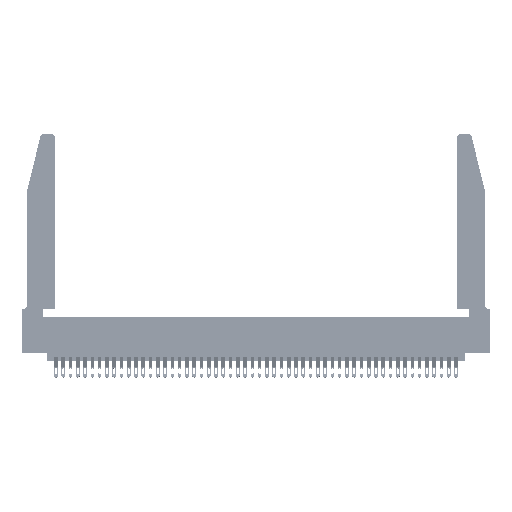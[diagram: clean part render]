
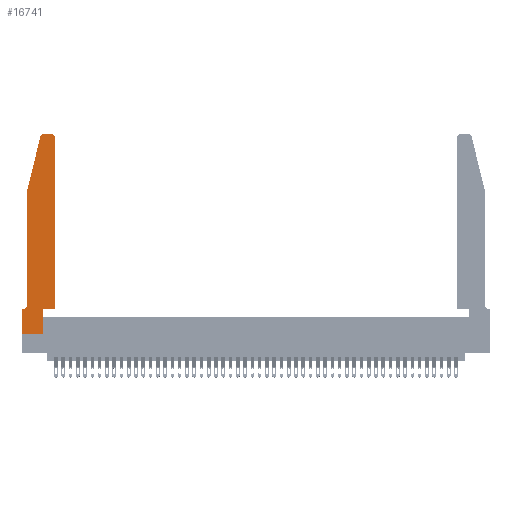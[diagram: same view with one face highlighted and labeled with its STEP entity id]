
A CAD part, top view. The second image highlights one B-rep face of the part: STEP entity #16741.
In plain terms, the highlighted planar face has unit normal (0, 0, 1).
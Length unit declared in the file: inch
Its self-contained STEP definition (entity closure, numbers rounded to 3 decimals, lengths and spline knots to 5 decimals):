
#298 = ORIENTED_EDGE ( 'NONE', *, *, #28404, .T. ) ;
#1066 = DIRECTION ( 'NONE',  ( 0., 0., -1. ) ) ;
#1741 = CARTESIAN_POINT ( 'NONE',  ( 0.0755, 2., 0.37 ) ) ;
#4132 = EDGE_CURVE ( 'NONE', #17867, #7614, #18595, .T. ) ;
#4492 = AXIS2_PLACEMENT_3D ( 'NONE', #38347, #20218, #45527 ) ;
#4777 = VECTOR ( 'NONE', #9166, 39.37008 ) ;
#5422 = CARTESIAN_POINT ( 'NONE',  ( 0.0755, 2., 0.37 ) ) ;
#5758 = LINE ( 'NONE', #1741, #31540 ) ;
#5837 = CIRCLE ( 'NONE', #22130, 0.03 ) ;
#6157 = EDGE_CURVE ( 'NONE', #44111, #42202, #5837, .T. ) ;
#6162 = DIRECTION ( 'NONE',  ( 1., 0., 0. ) ) ;
#6697 = ORIENTED_EDGE ( 'NONE', *, *, #16941, .T. ) ;
#7207 = CARTESIAN_POINT ( 'NONE',  ( 0.2605, 2.75, 0.37 ) ) ;
#7307 = CARTESIAN_POINT ( 'NONE',  ( 0., 0., 0.37 ) ) ;
#7614 = VERTEX_POINT ( 'NONE', #37270 ) ;
#7860 = VERTEX_POINT ( 'NONE', #38351 ) ;
#8932 = DIRECTION ( 'NONE',  ( 0., 1., 0. ) ) ;
#9166 = DIRECTION ( 'NONE',  ( -0.239, -0.971, 0. ) ) ;
#9358 = EDGE_CURVE ( 'NONE', #42269, #7860, #24771, .T. ) ;
#9392 = VECTOR ( 'NONE', #27850, 39.37008 ) ;
#13150 = CARTESIAN_POINT ( 'NONE',  ( 0.0755, 0.35, 0.37 ) ) ;
#13157 = VECTOR ( 'NONE', #36526, 39.37008 ) ;
#13175 = EDGE_CURVE ( 'NONE', #7614, #32033, #39189, .T. ) ;
#13488 = DIRECTION ( 'NONE',  ( 0., 0., 1. ) ) ;
#14235 = CARTESIAN_POINT ( 'NONE',  ( 0.2865, 0.35, 0.37 ) ) ;
#14913 = CIRCLE ( 'NONE', #44762, 0.03 ) ;
#15026 = VECTOR ( 'NONE', #28064, 39.37008 ) ;
#15258 = ORIENTED_EDGE ( 'NONE', *, *, #15825, .T. ) ;
#15629 = EDGE_CURVE ( 'NONE', #32033, #36441, #14913, .T. ) ;
#15825 = EDGE_CURVE ( 'NONE', #31957, #28430, #42158, .T. ) ;
#15850 = VECTOR ( 'NONE', #34772, 39.37008 ) ;
#15932 = VECTOR ( 'NONE', #18278, 39.37008 ) ;
#16144 = CARTESIAN_POINT ( 'NONE',  ( 0.4505, 0.35, 0.37 ) ) ;
#16468 = DIRECTION ( 'NONE',  ( 0., -1., 0. ) ) ;
#16524 = FACE_OUTER_BOUND ( 'NONE', #26219, .T. ) ;
#16741 = ADVANCED_FACE ( 'NONE', ( #16524 ), #34723, .T. ) ;
#16941 = EDGE_CURVE ( 'NONE', #36441, #44111, #17070, .T. ) ;
#17070 = LINE ( 'NONE', #7207, #15932 ) ;
#17366 = CARTESIAN_POINT ( 'NONE',  ( 0.25487, 2.72718, 0.37 ) ) ;
#17455 = CARTESIAN_POINT ( 'NONE',  ( 0.4205, 2.72, 0.37 ) ) ;
#17867 = VERTEX_POINT ( 'NONE', #14235 ) ;
#18144 = ORIENTED_EDGE ( 'NONE', *, *, #30583, .T. ) ;
#18278 = DIRECTION ( 'NONE',  ( -1., 0., 0. ) ) ;
#18595 = LINE ( 'NONE', #35418, #36829 ) ;
#18778 = ORIENTED_EDGE ( 'NONE', *, *, #34112, .T. ) ;
#19275 = VERTEX_POINT ( 'NONE', #33746 ) ;
#20218 = DIRECTION ( 'NONE',  ( 0., 0., 1. ) ) ;
#21123 = DIRECTION ( 'NONE',  ( 1., 0., 0. ) ) ;
#21349 = CARTESIAN_POINT ( 'NONE',  ( 0.0755, 0.42, 0.37 ) ) ;
#22130 = AXIS2_PLACEMENT_3D ( 'NONE', #35332, #13488, #38969 ) ;
#23169 = CARTESIAN_POINT ( 'NONE',  ( 0.0055, 0.42, 0.37 ) ) ;
#24318 = LINE ( 'NONE', #5422, #4777 ) ;
#24378 = CARTESIAN_POINT ( 'NONE',  ( 0.2865, 0.35, 0.37 ) ) ;
#24751 = ORIENTED_EDGE ( 'NONE', *, *, #13175, .T. ) ;
#24771 = CIRCLE ( 'NONE', #38357, 0.07 ) ;
#24934 = CARTESIAN_POINT ( 'NONE',  ( 0.4505, 2.72, 0.37 ) ) ;
#25608 = ORIENTED_EDGE ( 'NONE', *, *, #4132, .T. ) ;
#25919 = ORIENTED_EDGE ( 'NONE', *, *, #6157, .T. ) ;
#26219 = EDGE_LOOP ( 'NONE', ( #6697, #25919, #18778, #18144, #29362, #298, #32042, #15258, #43844, #25608, #24751, #38644 ) ) ;
#26834 = DIRECTION ( 'NONE',  ( -1., 0., 0. ) ) ;
#27850 = DIRECTION ( 'NONE',  ( -1., 0., 0. ) ) ;
#28012 = CARTESIAN_POINT ( 'NONE',  ( 0.2865, 0., 0.37 ) ) ;
#28064 = DIRECTION ( 'NONE',  ( 0., 1., 0. ) ) ;
#28147 = CARTESIAN_POINT ( 'NONE',  ( 0., 0., 0.37 ) ) ;
#28404 = EDGE_CURVE ( 'NONE', #7860, #32268, #39603, .T. ) ;
#28430 = VERTEX_POINT ( 'NONE', #28012 ) ;
#29362 = ORIENTED_EDGE ( 'NONE', *, *, #9358, .T. ) ;
#29533 = VECTOR ( 'NONE', #8932, 39.37008 ) ;
#30583 = EDGE_CURVE ( 'NONE', #19275, #42269, #5758, .T. ) ;
#31115 = CARTESIAN_POINT ( 'NONE',  ( 0., 0., 0.37 ) ) ;
#31540 = VECTOR ( 'NONE', #16468, 39.37008 ) ;
#31957 = VERTEX_POINT ( 'NONE', #28147 ) ;
#32033 = VERTEX_POINT ( 'NONE', #24934 ) ;
#32042 = ORIENTED_EDGE ( 'NONE', *, *, #33498, .T. ) ;
#32268 = VERTEX_POINT ( 'NONE', #33380 ) ;
#33380 = CARTESIAN_POINT ( 'NONE',  ( 0., 0.35, 0.37 ) ) ;
#33498 = EDGE_CURVE ( 'NONE', #32268, #31957, #35232, .T. ) ;
#33746 = CARTESIAN_POINT ( 'NONE',  ( 0.0755, 2., 0.37 ) ) ;
#34112 = EDGE_CURVE ( 'NONE', #42202, #19275, #24318, .T. ) ;
#34572 = CARTESIAN_POINT ( 'NONE',  ( 0.4205, 2.75, 0.37 ) ) ;
#34723 = PLANE ( 'NONE',  #4492 ) ;
#34772 = DIRECTION ( 'NONE',  ( 0., -1., 0. ) ) ;
#35232 = LINE ( 'NONE', #31115, #15850 ) ;
#35332 = CARTESIAN_POINT ( 'NONE',  ( 0.284, 2.72, 0.37 ) ) ;
#35418 = CARTESIAN_POINT ( 'NONE',  ( 0.4505, 0.35, 0.37 ) ) ;
#36441 = VERTEX_POINT ( 'NONE', #34572 ) ;
#36526 = DIRECTION ( 'NONE',  ( 1., 0., 0. ) ) ;
#36829 = VECTOR ( 'NONE', #6162, 39.37008 ) ;
#37270 = CARTESIAN_POINT ( 'NONE',  ( 0.4505, 0.35, 0.37 ) ) ;
#38347 = CARTESIAN_POINT ( 'NONE',  ( 0., 0.35, 0.37 ) ) ;
#38351 = CARTESIAN_POINT ( 'NONE',  ( 0.0055, 0.35, 0.37 ) ) ;
#38357 = AXIS2_PLACEMENT_3D ( 'NONE', #23169, #1066, #26834 ) ;
#38644 = ORIENTED_EDGE ( 'NONE', *, *, #15629, .T. ) ;
#38969 = DIRECTION ( 'NONE',  ( 1., 0., 0. ) ) ;
#39189 = LINE ( 'NONE', #16144, #29533 ) ;
#39603 = LINE ( 'NONE', #13150, #9392 ) ;
#42158 = LINE ( 'NONE', #7307, #13157 ) ;
#42202 = VERTEX_POINT ( 'NONE', #17366 ) ;
#42269 = VERTEX_POINT ( 'NONE', #21349 ) ;
#42820 = DIRECTION ( 'NONE',  ( 0., 0., 1. ) ) ;
#43844 = ORIENTED_EDGE ( 'NONE', *, *, #44880, .T. ) ;
#43955 = LINE ( 'NONE', #24378, #15026 ) ;
#44111 = VERTEX_POINT ( 'NONE', #45999 ) ;
#44762 = AXIS2_PLACEMENT_3D ( 'NONE', #17455, #42820, #21123 ) ;
#44880 = EDGE_CURVE ( 'NONE', #28430, #17867, #43955, .T. ) ;
#45527 = DIRECTION ( 'NONE',  ( 1., 0., 0. ) ) ;
#45999 = CARTESIAN_POINT ( 'NONE',  ( 0.284, 2.75, 0.37 ) ) ;
